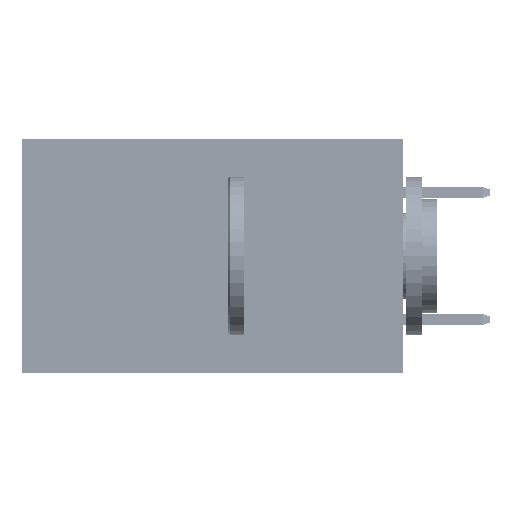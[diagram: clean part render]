
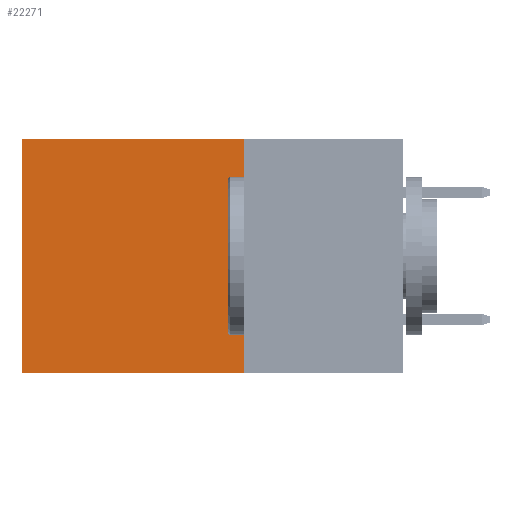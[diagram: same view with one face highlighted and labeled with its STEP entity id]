
A CAD part, left-side view. The second image highlights one B-rep face of the part: STEP entity #22271.
In plain terms, the highlighted planar face has unit normal (-1, 0, 0).
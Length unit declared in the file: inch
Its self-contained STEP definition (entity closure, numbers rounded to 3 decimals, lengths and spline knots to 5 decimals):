
#559 = ORIENTED_EDGE ( 'NONE', *, *, #32208, .T. ) ;
#796 = ORIENTED_EDGE ( 'NONE', *, *, #48255, .T. ) ;
#2826 = PLANE ( 'NONE',  #7760 ) ;
#3068 = DIRECTION ( 'NONE',  ( 0., 1., 0. ) ) ;
#5895 = LINE ( 'NONE', #6881, #23551 ) ;
#6130 = DIRECTION ( 'NONE',  ( 0., 0., -1. ) ) ;
#6375 = CARTESIAN_POINT ( 'NONE',  ( 0.2875, 0.6, -0.37 ) ) ;
#6623 = FACE_OUTER_BOUND ( 'NONE', #39012, .T. ) ;
#6881 = CARTESIAN_POINT ( 'NONE',  ( 0.2875, 0.25, 0. ) ) ;
#7248 = ORIENTED_EDGE ( 'NONE', *, *, #20315, .F. ) ;
#7760 = AXIS2_PLACEMENT_3D ( 'NONE', #18255, #42216, #19176 ) ;
#10994 = CARTESIAN_POINT ( 'NONE',  ( 0.2875, 0.6, 0. ) ) ;
#12175 = VERTEX_POINT ( 'NONE', #18120 ) ;
#13981 = LINE ( 'NONE', #17754, #47809 ) ;
#15815 = LINE ( 'NONE', #34860, #40738 ) ;
#17754 = CARTESIAN_POINT ( 'NONE',  ( 0.2875, 0.25, 0. ) ) ;
#18120 = CARTESIAN_POINT ( 'NONE',  ( 0.2875, 0.25, 0. ) ) ;
#18255 = CARTESIAN_POINT ( 'NONE',  ( 0.2875, 0.25, 0. ) ) ;
#19176 = DIRECTION ( 'NONE',  ( 0., 0., -1. ) ) ;
#20099 = CARTESIAN_POINT ( 'NONE',  ( 0.2875, 0.25, -0.37 ) ) ;
#20315 = EDGE_CURVE ( 'NONE', #12175, #27663, #5895, .T. ) ;
#21558 = ORIENTED_EDGE ( 'NONE', *, *, #48355, .F. ) ;
#22271 = ADVANCED_FACE ( 'NONE', ( #6623 ), #2826, .F. ) ;
#23400 = DIRECTION ( 'NONE',  ( 0., 0., -1. ) ) ;
#23551 = VECTOR ( 'NONE', #6130, 39.37008 ) ;
#24892 = CARTESIAN_POINT ( 'NONE',  ( 0.2875, 0.25, -0.37 ) ) ;
#27663 = VERTEX_POINT ( 'NONE', #24892 ) ;
#32208 = EDGE_CURVE ( 'NONE', #12175, #39704, #13981, .T. ) ;
#33742 = VERTEX_POINT ( 'NONE', #6375 ) ;
#34860 = CARTESIAN_POINT ( 'NONE',  ( 0.2875, 0.6, 0. ) ) ;
#36535 = DIRECTION ( 'NONE',  ( 0., 1., 0. ) ) ;
#39012 = EDGE_LOOP ( 'NONE', ( #796, #21558, #7248, #559 ) ) ;
#39091 = VECTOR ( 'NONE', #36535, 39.37008 ) ;
#39704 = VERTEX_POINT ( 'NONE', #10994 ) ;
#40738 = VECTOR ( 'NONE', #23400, 39.37008 ) ;
#42216 = DIRECTION ( 'NONE',  ( 1., 0., 0. ) ) ;
#44117 = LINE ( 'NONE', #20099, #39091 ) ;
#47809 = VECTOR ( 'NONE', #3068, 39.37008 ) ;
#48255 = EDGE_CURVE ( 'NONE', #39704, #33742, #15815, .T. ) ;
#48355 = EDGE_CURVE ( 'NONE', #27663, #33742, #44117, .T. ) ;
